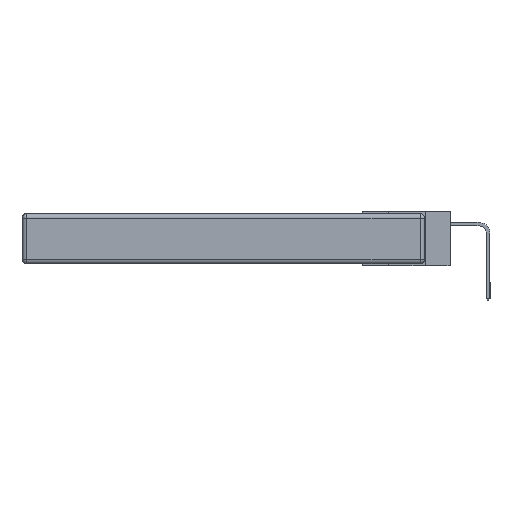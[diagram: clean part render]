
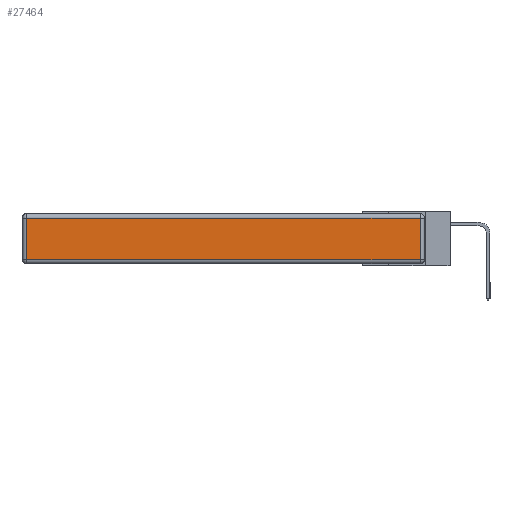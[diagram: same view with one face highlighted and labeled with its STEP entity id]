
A CAD part, left-side view. The second image highlights one B-rep face of the part: STEP entity #27464.
In plain terms, the highlighted planar face has unit normal (-1, 0, 0).
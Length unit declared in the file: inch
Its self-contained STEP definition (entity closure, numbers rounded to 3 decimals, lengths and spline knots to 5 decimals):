
#231 = EDGE_CURVE ( 'NONE', #12480, #6196, #15266, .T. ) ;
#363 = CARTESIAN_POINT ( 'NONE',  ( 0., 0.03, -0.03 ) ) ;
#1981 = DIRECTION ( 'NONE',  ( 0., 0., -1. ) ) ;
#2716 = EDGE_CURVE ( 'NONE', #3360, #12480, #25905, .T. ) ;
#3166 = DIRECTION ( 'NONE',  ( 0., 1., 0. ) ) ;
#3360 = VERTEX_POINT ( 'NONE', #15769 ) ;
#4249 = ORIENTED_EDGE ( 'NONE', *, *, #231, .T. ) ;
#6196 = VERTEX_POINT ( 'NONE', #28591 ) ;
#6290 = DIRECTION ( 'NONE',  ( 0., 0., 1. ) ) ;
#8257 = PLANE ( 'NONE',  #12086 ) ;
#8566 = CARTESIAN_POINT ( 'NONE',  ( 0., 0., -0.343 ) ) ;
#9354 = VECTOR ( 'NONE', #3166, 39.37008 ) ;
#12086 = AXIS2_PLACEMENT_3D ( 'NONE', #8566, #23282, #28127 ) ;
#12107 = EDGE_CURVE ( 'NONE', #26287, #3360, #18911, .T. ) ;
#12480 = VERTEX_POINT ( 'NONE', #363 ) ;
#12956 = EDGE_CURVE ( 'NONE', #6196, #26287, #13391, .T. ) ;
#12986 = VECTOR ( 'NONE', #1981, 39.37008 ) ;
#13391 = LINE ( 'NONE', #17000, #12986 ) ;
#15266 = LINE ( 'NONE', #18070, #9354 ) ;
#15350 = ORIENTED_EDGE ( 'NONE', *, *, #12107, .T. ) ;
#15438 = ORIENTED_EDGE ( 'NONE', *, *, #12956, .T. ) ;
#15769 = CARTESIAN_POINT ( 'NONE',  ( 0., 0.03, -0.313 ) ) ;
#16154 = FACE_OUTER_BOUND ( 'NONE', #30025, .T. ) ;
#17000 = CARTESIAN_POINT ( 'NONE',  ( 0., 2.72, -0.343 ) ) ;
#17815 = VECTOR ( 'NONE', #6290, 39.37008 ) ;
#18070 = CARTESIAN_POINT ( 'NONE',  ( 0., 2.75, -0.03 ) ) ;
#18911 = LINE ( 'NONE', #25064, #21225 ) ;
#21225 = VECTOR ( 'NONE', #32194, 39.37008 ) ;
#21705 = ORIENTED_EDGE ( 'NONE', *, *, #2716, .T. ) ;
#23282 = DIRECTION ( 'NONE',  ( -1., 0., 0. ) ) ;
#25064 = CARTESIAN_POINT ( 'NONE',  ( 0., 0., -0.313 ) ) ;
#25497 = CARTESIAN_POINT ( 'NONE',  ( 0., 2.72, -0.313 ) ) ;
#25905 = LINE ( 'NONE', #31603, #17815 ) ;
#26287 = VERTEX_POINT ( 'NONE', #25497 ) ;
#27464 = ADVANCED_FACE ( 'NONE', ( #16154 ), #8257, .T. ) ;
#28127 = DIRECTION ( 'NONE',  ( 0., 0., 1. ) ) ;
#28591 = CARTESIAN_POINT ( 'NONE',  ( 0., 2.72, -0.03 ) ) ;
#30025 = EDGE_LOOP ( 'NONE', ( #15350, #21705, #4249, #15438 ) ) ;
#31603 = CARTESIAN_POINT ( 'NONE',  ( 0., 0.03, -0.343 ) ) ;
#32194 = DIRECTION ( 'NONE',  ( 0., -1., 0. ) ) ;
